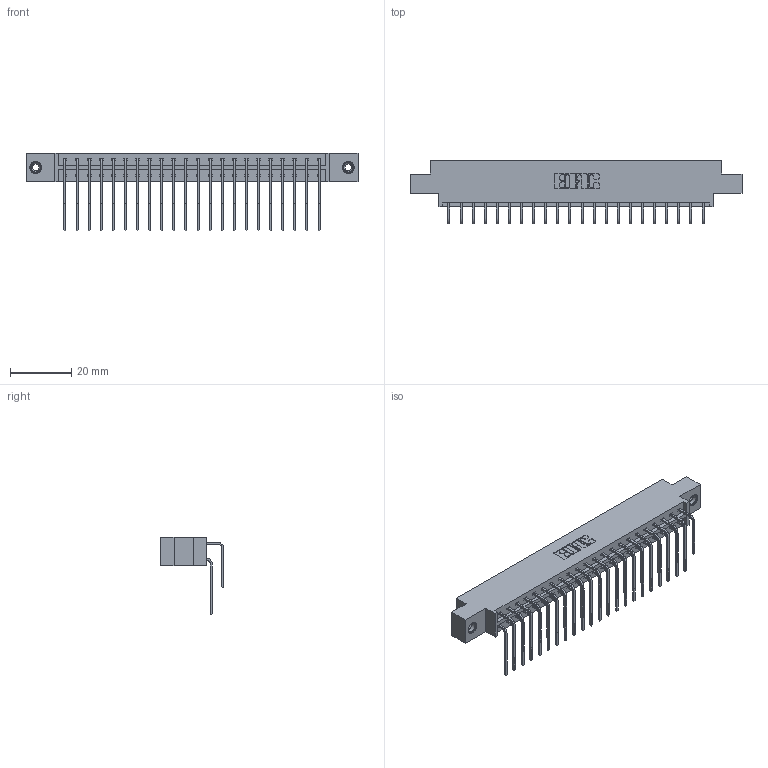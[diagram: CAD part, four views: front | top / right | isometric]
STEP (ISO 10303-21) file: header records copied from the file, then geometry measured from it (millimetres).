
FILE_DESCRIPTION (( 'STEP AP203' ), '1' );
FILE_NAME ('333-044-559-808.STEP', '2018-08-03T21:48:14', ( '' ), ( '' ), 'SwSTEP 2.0', 'SolidWorks 2016', '' );
FILE_SCHEMA (( 'CONFIG_CONTROL_DESIGN' ));
Length unit declared in the file: inch
Products named in the file (5): 333 Part_Offset - .156 Dia - TI; 345-292-001_558 559 Tail - 1; 345-292-001_559 Tail - 2; 345-250-001_345-250-003-102; 333-044-559-808
Assembly tree (47 placements, depth 2):
  333-044-559-808
    333 Part_Offset - .156 Dia - TI
    345-292-001_558 559 Tail - 1  x22
    345-292-001_559 Tail - 2  x22
    345-250-001_345-250-003-102  x2
Bounding box: 108.71 x 20.9 x 25.53 mm (x, y, z)
Volume: 10931.4 mm3; surface area: 14215.6 mm2
Topology: 47 solids, 47 shells, 2554 faces, 7543 edges, 4962 vertices
Faces by surface type: plane 1778, cylinder 760, cone 12, torus 4
Entity records: 19842 total; most frequent: CARTESIAN_POINT 3348, ORIENTED_EDGE 3226, DIRECTION 2907, EDGE_CURVE 1613, VECTOR 1425, LINE 1425, VERTEX_POINT 1068, AXIS2_PLACEMENT_3D 741
